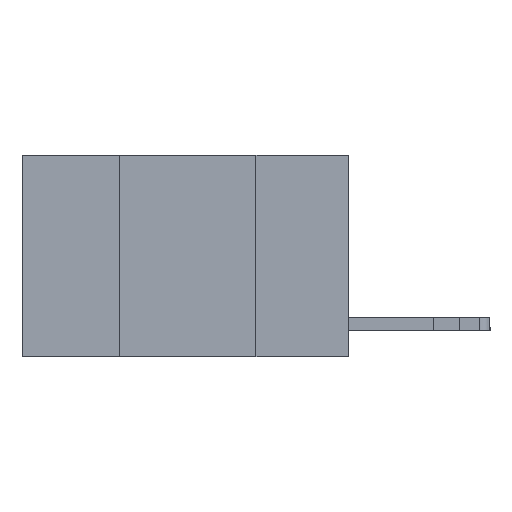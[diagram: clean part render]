
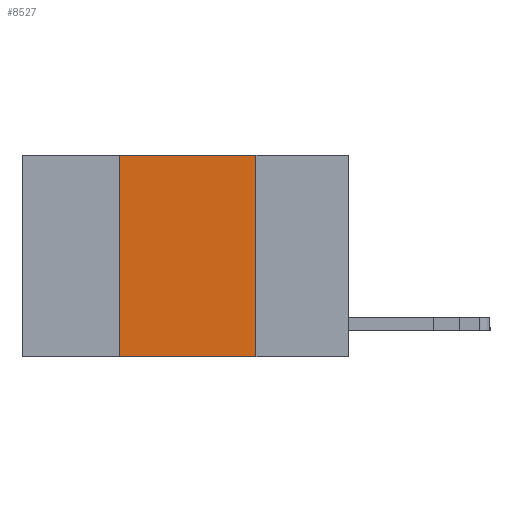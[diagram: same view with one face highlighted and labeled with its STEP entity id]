
A CAD part, left-side view. The second image highlights one B-rep face of the part: STEP entity #8527.
In plain terms, the highlighted planar face has unit normal (-1, 0, 0).
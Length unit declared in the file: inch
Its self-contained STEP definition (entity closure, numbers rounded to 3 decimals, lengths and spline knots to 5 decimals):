
#20 = LINE ( 'NONE', #3890, #8904 ) ;
#233 = ORIENTED_EDGE ( 'NONE', *, *, #525, .F. ) ;
#432 = CARTESIAN_POINT ( 'NONE',  ( 0., 0.17, -0.37 ) ) ;
#438 = EDGE_CURVE ( 'NONE', #12251, #9832, #12384, .T. ) ;
#525 = EDGE_CURVE ( 'NONE', #703, #7256, #20, .T. ) ;
#703 = VERTEX_POINT ( 'NONE', #12125 ) ;
#708 = EDGE_LOOP ( 'NONE', ( #4449, #1984, #233, #1720 ) ) ;
#1251 = DIRECTION ( 'NONE',  ( 0., -1., 0. ) ) ;
#1311 = CARTESIAN_POINT ( 'NONE',  ( 0., 0.42, 0. ) ) ;
#1500 = DIRECTION ( 'NONE',  ( 0., -1., 0. ) ) ;
#1640 = VECTOR ( 'NONE', #8579, 39.37008 ) ;
#1720 = ORIENTED_EDGE ( 'NONE', *, *, #2783, .T. ) ;
#1889 = VECTOR ( 'NONE', #1251, 39.37008 ) ;
#1984 = ORIENTED_EDGE ( 'NONE', *, *, #10163, .F. ) ;
#2266 = CARTESIAN_POINT ( 'NONE',  ( 0., 0.6, 0. ) ) ;
#2783 = EDGE_CURVE ( 'NONE', #703, #9832, #6143, .T. ) ;
#3808 = PLANE ( 'NONE',  #4516 ) ;
#3890 = CARTESIAN_POINT ( 'NONE',  ( 0., 0.42, 0. ) ) ;
#4126 = CARTESIAN_POINT ( 'NONE',  ( 0., 0.17, 0. ) ) ;
#4449 = ORIENTED_EDGE ( 'NONE', *, *, #438, .F. ) ;
#4516 = AXIS2_PLACEMENT_3D ( 'NONE', #10656, #4692, #10590 ) ;
#4692 = DIRECTION ( 'NONE',  ( 1., 0., 0. ) ) ;
#6143 = LINE ( 'NONE', #10185, #8792 ) ;
#7256 = VERTEX_POINT ( 'NONE', #1311 ) ;
#7768 = DIRECTION ( 'NONE',  ( 0., 0., 1. ) ) ;
#8527 = ADVANCED_FACE ( 'NONE', ( #8619 ), #3808, .F. ) ;
#8579 = DIRECTION ( 'NONE',  ( 0., 0., -1. ) ) ;
#8619 = FACE_OUTER_BOUND ( 'NONE', #708, .T. ) ;
#8710 = CARTESIAN_POINT ( 'NONE',  ( 0., 0.17, 0. ) ) ;
#8792 = VECTOR ( 'NONE', #1500, 39.37008 ) ;
#8904 = VECTOR ( 'NONE', #7768, 39.37008 ) ;
#9047 = LINE ( 'NONE', #2266, #1889 ) ;
#9832 = VERTEX_POINT ( 'NONE', #432 ) ;
#10163 = EDGE_CURVE ( 'NONE', #7256, #12251, #9047, .T. ) ;
#10185 = CARTESIAN_POINT ( 'NONE',  ( 0., 0.6, -0.37 ) ) ;
#10590 = DIRECTION ( 'NONE',  ( 0., 0., -1. ) ) ;
#10656 = CARTESIAN_POINT ( 'NONE',  ( 0., 0.6, 0. ) ) ;
#12125 = CARTESIAN_POINT ( 'NONE',  ( 0., 0.42, -0.37 ) ) ;
#12251 = VERTEX_POINT ( 'NONE', #4126 ) ;
#12384 = LINE ( 'NONE', #8710, #1640 ) ;
